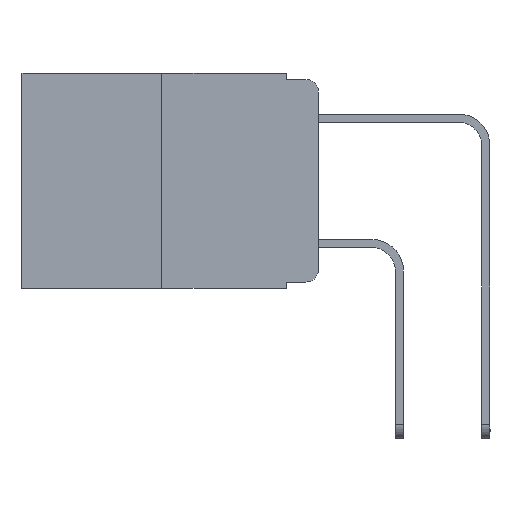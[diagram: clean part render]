
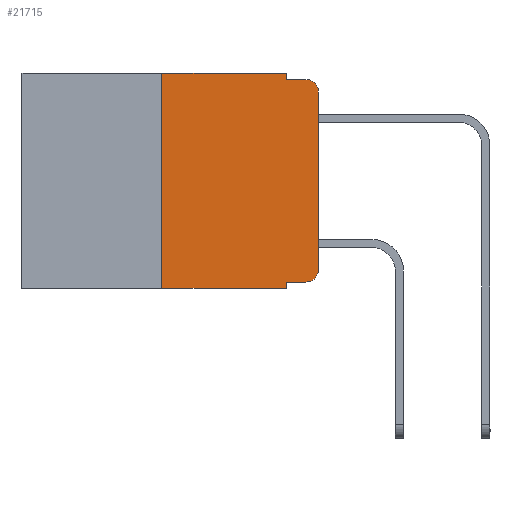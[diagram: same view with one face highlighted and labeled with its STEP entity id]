
A CAD part, left-side view. The second image highlights one B-rep face of the part: STEP entity #21715.
In plain terms, the highlighted planar face has unit normal (-1, 0, 0).
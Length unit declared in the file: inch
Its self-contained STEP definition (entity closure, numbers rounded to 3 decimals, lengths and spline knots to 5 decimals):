
#147 = EDGE_CURVE ( 'NONE', #5992, #4949, #10132, .T. ) ;
#214 = DIRECTION ( 'NONE',  ( 0., -1., 0. ) ) ;
#281 = VECTOR ( 'NONE', #19098, 39.37008 ) ;
#1060 = VERTEX_POINT ( 'NONE', #1465 ) ;
#1195 = ORIENTED_EDGE ( 'NONE', *, *, #2586, .F. ) ;
#1375 = CARTESIAN_POINT ( 'NONE',  ( 0., 0., -0.03 ) ) ;
#1443 = DIRECTION ( 'NONE',  ( 0., 0., -1. ) ) ;
#1465 = CARTESIAN_POINT ( 'NONE',  ( 0., 0.051, -0.01 ) ) ;
#1545 = EDGE_CURVE ( 'NONE', #22225, #26181, #23160, .T. ) ;
#1674 = ORIENTED_EDGE ( 'NONE', *, *, #3224, .T. ) ;
#2323 = CARTESIAN_POINT ( 'NONE',  ( 0., 0.473, -0.343 ) ) ;
#2440 = CARTESIAN_POINT ( 'NONE',  ( 0., 0.25, -0.343 ) ) ;
#2519 = LINE ( 'NONE', #25588, #24901 ) ;
#2586 = EDGE_CURVE ( 'NONE', #1060, #12380, #28242, .T. ) ;
#3048 = CARTESIAN_POINT ( 'NONE',  ( 0., 0.02, -0.01 ) ) ;
#3099 = VERTEX_POINT ( 'NONE', #17192 ) ;
#3224 = EDGE_CURVE ( 'NONE', #26181, #8278, #4402, .T. ) ;
#3934 = AXIS2_PLACEMENT_3D ( 'NONE', #19433, #8711, #24040 ) ;
#4143 = CARTESIAN_POINT ( 'NONE',  ( 0., 0.473, 0. ) ) ;
#4166 = DIRECTION ( 'NONE',  ( 0., -1., 0. ) ) ;
#4179 = CARTESIAN_POINT ( 'NONE',  ( 0., 0.25, 0. ) ) ;
#4402 = LINE ( 'NONE', #12447, #281 ) ;
#4949 = VERTEX_POINT ( 'NONE', #4179 ) ;
#5038 = EDGE_CURVE ( 'NONE', #8034, #1060, #2519, .T. ) ;
#5992 = VERTEX_POINT ( 'NONE', #2440 ) ;
#7410 = CARTESIAN_POINT ( 'NONE',  ( 0., 0.051, -0.333 ) ) ;
#7501 = FACE_OUTER_BOUND ( 'NONE', #10830, .T. ) ;
#8034 = VERTEX_POINT ( 'NONE', #28088 ) ;
#8278 = VERTEX_POINT ( 'NONE', #1375 ) ;
#8711 = DIRECTION ( 'NONE',  ( -1., 0., 0. ) ) ;
#9054 = ORIENTED_EDGE ( 'NONE', *, *, #147, .F. ) ;
#9231 = ORIENTED_EDGE ( 'NONE', *, *, #17997, .F. ) ;
#10078 = LINE ( 'NONE', #27096, #11474 ) ;
#10132 = LINE ( 'NONE', #13814, #10499 ) ;
#10499 = VECTOR ( 'NONE', #24674, 39.37008 ) ;
#10830 = EDGE_LOOP ( 'NONE', ( #1674, #17259, #1195, #17548, #9231, #9054, #11837, #28406, #20075, #19584 ) ) ;
#11185 = CARTESIAN_POINT ( 'NONE',  ( 0., 0., -0.313 ) ) ;
#11474 = VECTOR ( 'NONE', #17949, 39.37008 ) ;
#11828 = CIRCLE ( 'NONE', #3934, 0.02 ) ;
#11837 = ORIENTED_EDGE ( 'NONE', *, *, #17891, .T. ) ;
#12380 = VERTEX_POINT ( 'NONE', #3048 ) ;
#12394 = VECTOR ( 'NONE', #4166, 39.37008 ) ;
#12447 = CARTESIAN_POINT ( 'NONE',  ( 0., 0., 0. ) ) ;
#12475 = LINE ( 'NONE', #2323, #25569 ) ;
#13237 = DIRECTION ( 'NONE',  ( 0., -1., 0. ) ) ;
#13504 = EDGE_CURVE ( 'NONE', #8278, #12380, #11828, .T. ) ;
#13513 = LINE ( 'NONE', #17560, #24529 ) ;
#13814 = CARTESIAN_POINT ( 'NONE',  ( 0., 0.25, 0. ) ) ;
#15425 = CARTESIAN_POINT ( 'NONE',  ( 0., 0.02, -0.313 ) ) ;
#15916 = DIRECTION ( 'NONE',  ( 0., -1., 0. ) ) ;
#16299 = EDGE_CURVE ( 'NONE', #22666, #22225, #22905, .T. ) ;
#16814 = CARTESIAN_POINT ( 'NONE',  ( 0., 0.051, -0.333 ) ) ;
#17192 = CARTESIAN_POINT ( 'NONE',  ( 0., 0.051, -0.343 ) ) ;
#17259 = ORIENTED_EDGE ( 'NONE', *, *, #13504, .T. ) ;
#17328 = CARTESIAN_POINT ( 'NONE',  ( 0., 0.02, -0.333 ) ) ;
#17436 = EDGE_CURVE ( 'NONE', #22666, #3099, #10078, .T. ) ;
#17544 = DIRECTION ( 'NONE',  ( -1., 0., 0. ) ) ;
#17548 = ORIENTED_EDGE ( 'NONE', *, *, #5038, .F. ) ;
#17560 = CARTESIAN_POINT ( 'NONE',  ( 0., 0.473, 0. ) ) ;
#17891 = EDGE_CURVE ( 'NONE', #5992, #3099, #12475, .T. ) ;
#17949 = DIRECTION ( 'NONE',  ( 0., 0., -1. ) ) ;
#17997 = EDGE_CURVE ( 'NONE', #4949, #8034, #13513, .T. ) ;
#18088 = VECTOR ( 'NONE', #15916, 39.37008 ) ;
#19098 = DIRECTION ( 'NONE',  ( 0., 0., 1. ) ) ;
#19433 = CARTESIAN_POINT ( 'NONE',  ( 0., 0.02, -0.03 ) ) ;
#19482 = DIRECTION ( 'NONE',  ( 1., 0., 0. ) ) ;
#19579 = DIRECTION ( 'NONE',  ( 0., 0., -1. ) ) ;
#19584 = ORIENTED_EDGE ( 'NONE', *, *, #1545, .T. ) ;
#19660 = DIRECTION ( 'NONE',  ( 0., 0., -1. ) ) ;
#19977 = CARTESIAN_POINT ( 'NONE',  ( 0., 0.051, -0.01 ) ) ;
#20075 = ORIENTED_EDGE ( 'NONE', *, *, #16299, .T. ) ;
#20708 = AXIS2_PLACEMENT_3D ( 'NONE', #4143, #19482, #19579 ) ;
#21715 = ADVANCED_FACE ( 'NONE', ( #7501 ), #28229, .F. ) ;
#22225 = VERTEX_POINT ( 'NONE', #17328 ) ;
#22666 = VERTEX_POINT ( 'NONE', #16814 ) ;
#22905 = LINE ( 'NONE', #7410, #18088 ) ;
#23160 = CIRCLE ( 'NONE', #27112, 0.02 ) ;
#24040 = DIRECTION ( 'NONE',  ( 0., 0., -1. ) ) ;
#24529 = VECTOR ( 'NONE', #13237, 39.37008 ) ;
#24674 = DIRECTION ( 'NONE',  ( 0., 0., 1. ) ) ;
#24901 = VECTOR ( 'NONE', #1443, 39.37008 ) ;
#25569 = VECTOR ( 'NONE', #214, 39.37008 ) ;
#25588 = CARTESIAN_POINT ( 'NONE',  ( 0., 0.051, 0. ) ) ;
#26181 = VERTEX_POINT ( 'NONE', #11185 ) ;
#27096 = CARTESIAN_POINT ( 'NONE',  ( 0., 0.051, 0. ) ) ;
#27112 = AXIS2_PLACEMENT_3D ( 'NONE', #15425, #17544, #19660 ) ;
#28088 = CARTESIAN_POINT ( 'NONE',  ( 0., 0.051, 0. ) ) ;
#28229 = PLANE ( 'NONE',  #20708 ) ;
#28242 = LINE ( 'NONE', #19977, #12394 ) ;
#28406 = ORIENTED_EDGE ( 'NONE', *, *, #17436, .F. ) ;
